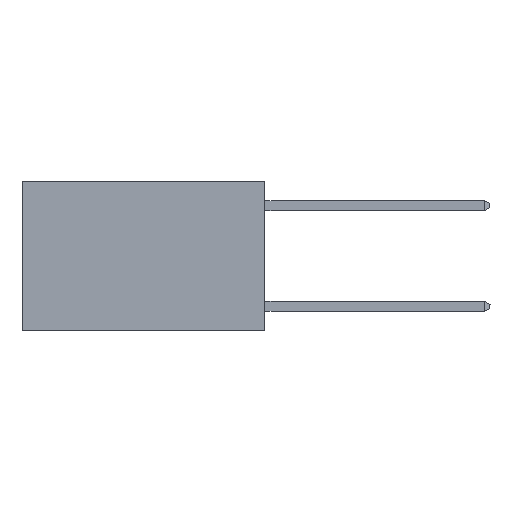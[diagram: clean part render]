
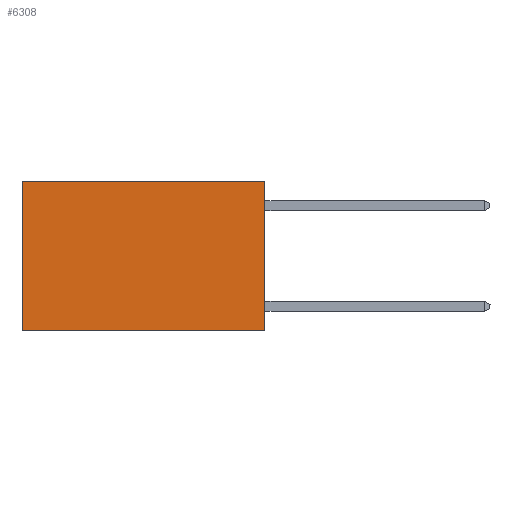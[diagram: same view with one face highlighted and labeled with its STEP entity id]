
A CAD part, left-side view. The second image highlights one B-rep face of the part: STEP entity #6308.
In plain terms, the highlighted planar face has unit normal (-1, 0, 0).
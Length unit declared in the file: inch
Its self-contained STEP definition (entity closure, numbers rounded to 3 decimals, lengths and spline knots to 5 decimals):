
#218 = DIRECTION ( 'NONE',  ( 0., 1., 0. ) ) ;
#828 = CARTESIAN_POINT ( 'NONE',  ( 0.2625, 0., -0.37 ) ) ;
#1366 = DIRECTION ( 'NONE',  ( 1., 0., 0. ) ) ;
#1539 = CARTESIAN_POINT ( 'NONE',  ( 0.2625, 0.6, 0. ) ) ;
#1786 = VERTEX_POINT ( 'NONE', #5603 ) ;
#2031 = EDGE_CURVE ( 'NONE', #4803, #3324, #9375, .T. ) ;
#2789 = VECTOR ( 'NONE', #218, 39.37008 ) ;
#2862 = VECTOR ( 'NONE', #13694, 39.37008 ) ;
#3324 = VERTEX_POINT ( 'NONE', #13267 ) ;
#3807 = LINE ( 'NONE', #4247, #6152 ) ;
#4247 = CARTESIAN_POINT ( 'NONE',  ( 0.2625, 0., 0. ) ) ;
#4302 = DIRECTION ( 'NONE',  ( 0., 0., -1. ) ) ;
#4322 = ORIENTED_EDGE ( 'NONE', *, *, #11156, .T. ) ;
#4479 = PLANE ( 'NONE',  #9334 ) ;
#4803 = VERTEX_POINT ( 'NONE', #1539 ) ;
#5603 = CARTESIAN_POINT ( 'NONE',  ( 0.2625, 0., 0. ) ) ;
#5642 = CARTESIAN_POINT ( 'NONE',  ( 0.2625, 0., 0. ) ) ;
#5842 = DIRECTION ( 'NONE',  ( 0., 0., -1. ) ) ;
#6152 = VECTOR ( 'NONE', #4302, 39.37008 ) ;
#6308 = ADVANCED_FACE ( 'NONE', ( #7250 ), #4479, .F. ) ;
#6675 = LINE ( 'NONE', #10484, #2862 ) ;
#7084 = LINE ( 'NONE', #9769, #2789 ) ;
#7110 = ORIENTED_EDGE ( 'NONE', *, *, #8838, .F. ) ;
#7250 = FACE_OUTER_BOUND ( 'NONE', #9631, .T. ) ;
#8838 = EDGE_CURVE ( 'NONE', #10065, #3324, #6675, .T. ) ;
#9191 = VECTOR ( 'NONE', #5842, 39.37008 ) ;
#9334 = AXIS2_PLACEMENT_3D ( 'NONE', #5642, #1366, #10842 ) ;
#9375 = LINE ( 'NONE', #13244, #9191 ) ;
#9616 = EDGE_CURVE ( 'NONE', #1786, #10065, #3807, .T. ) ;
#9631 = EDGE_LOOP ( 'NONE', ( #11615, #7110, #13570, #4322 ) ) ;
#9769 = CARTESIAN_POINT ( 'NONE',  ( 0.2625, 0., 0. ) ) ;
#10065 = VERTEX_POINT ( 'NONE', #828 ) ;
#10484 = CARTESIAN_POINT ( 'NONE',  ( 0.2625, 0., -0.37 ) ) ;
#10842 = DIRECTION ( 'NONE',  ( 0., 0., -1. ) ) ;
#11156 = EDGE_CURVE ( 'NONE', #1786, #4803, #7084, .T. ) ;
#11615 = ORIENTED_EDGE ( 'NONE', *, *, #2031, .T. ) ;
#13244 = CARTESIAN_POINT ( 'NONE',  ( 0.2625, 0.6, 0. ) ) ;
#13267 = CARTESIAN_POINT ( 'NONE',  ( 0.2625, 0.6, -0.37 ) ) ;
#13570 = ORIENTED_EDGE ( 'NONE', *, *, #9616, .F. ) ;
#13694 = DIRECTION ( 'NONE',  ( 0., 1., 0. ) ) ;
